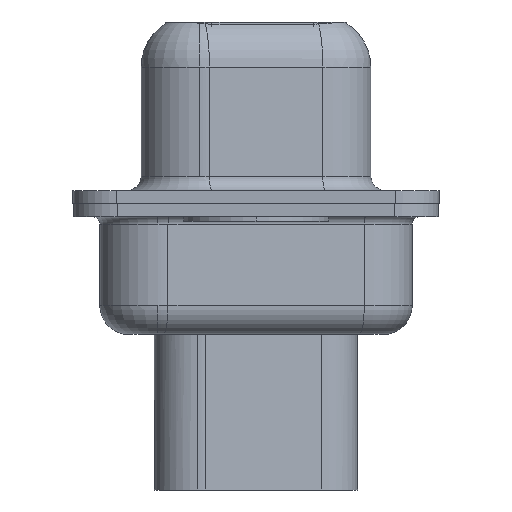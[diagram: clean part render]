
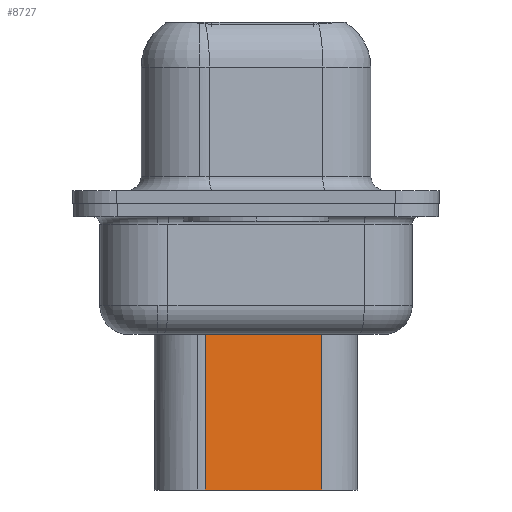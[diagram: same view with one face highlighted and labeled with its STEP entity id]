
A CAD part, left-side view. The second image highlights one B-rep face of the part: STEP entity #8727.
In plain terms, the highlighted planar face has unit normal (-0.985, -0.174, 0).
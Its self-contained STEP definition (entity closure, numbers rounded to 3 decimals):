
#24 = VERTEX_POINT ( 'NONE', #567 ) ;
#262 = AXIS2_PLACEMENT_3D ( 'NONE', #1603, #4441, #6333 ) ;
#567 = CARTESIAN_POINT ( 'NONE',  ( 5.224, -2.26, -9.85 ) ) ;
#669 = LINE ( 'NONE', #8529, #1882 ) ;
#914 = EDGE_CURVE ( 'NONE', #2439, #7228, #5295, .T. ) ;
#1603 = CARTESIAN_POINT ( 'NONE',  ( 4.519, 1.74, -3.1 ) ) ;
#1882 = VECTOR ( 'NONE', #12528, 1000. ) ;
#2271 = EDGE_LOOP ( 'NONE', ( #5961, #12387, #9970, #8436 ) ) ;
#2317 = VECTOR ( 'NONE', #2833, 1000. ) ;
#2439 = VERTEX_POINT ( 'NONE', #3637 ) ;
#2833 = DIRECTION ( 'NONE',  ( 0., 0., -1. ) ) ;
#3376 = DIRECTION ( 'NONE',  ( -0.174, 0.985, 0. ) ) ;
#3637 = CARTESIAN_POINT ( 'NONE',  ( 5.224, -2.26, -3.975 ) ) ;
#4441 = DIRECTION ( 'NONE',  ( -0.985, -0.174, 0. ) ) ;
#4583 = VECTOR ( 'NONE', #3376, 1000. ) ;
#5295 = LINE ( 'NONE', #10312, #4583 ) ;
#5961 = ORIENTED_EDGE ( 'NONE', *, *, #12231, .F. ) ;
#6079 = EDGE_CURVE ( 'NONE', #24, #10678, #11180, .T. ) ;
#6113 = EDGE_CURVE ( 'NONE', #7228, #10678, #9459, .T. ) ;
#6333 = DIRECTION ( 'NONE',  ( 0.174, -0.985, 0. ) ) ;
#7228 = VERTEX_POINT ( 'NONE', #12945 ) ;
#7294 = DIRECTION ( 'NONE',  ( -0.174, 0.985, 0. ) ) ;
#8436 = ORIENTED_EDGE ( 'NONE', *, *, #6079, .F. ) ;
#8529 = CARTESIAN_POINT ( 'NONE',  ( 5.224, -2.26, -3.1 ) ) ;
#8727 = ADVANCED_FACE ( 'NONE', ( #10516 ), #10446, .T. ) ;
#9459 = LINE ( 'NONE', #12720, #2317 ) ;
#9967 = CARTESIAN_POINT ( 'NONE',  ( 4.519, 1.74, -9.85 ) ) ;
#9970 = ORIENTED_EDGE ( 'NONE', *, *, #6113, .T. ) ;
#10312 = CARTESIAN_POINT ( 'NONE',  ( 4.348, 2.709, -3.975 ) ) ;
#10446 = PLANE ( 'NONE',  #262 ) ;
#10471 = VECTOR ( 'NONE', #7294, 1000. ) ;
#10516 = FACE_OUTER_BOUND ( 'NONE', #2271, .T. ) ;
#10678 = VERTEX_POINT ( 'NONE', #9967 ) ;
#11180 = LINE ( 'NONE', #12344, #10471 ) ;
#12231 = EDGE_CURVE ( 'NONE', #2439, #24, #669, .T. ) ;
#12344 = CARTESIAN_POINT ( 'NONE',  ( 4.519, 1.74, -9.85 ) ) ;
#12387 = ORIENTED_EDGE ( 'NONE', *, *, #914, .T. ) ;
#12528 = DIRECTION ( 'NONE',  ( 0., 0., -1. ) ) ;
#12720 = CARTESIAN_POINT ( 'NONE',  ( 4.519, 1.74, -3.1 ) ) ;
#12945 = CARTESIAN_POINT ( 'NONE',  ( 4.519, 1.74, -3.975 ) ) ;
